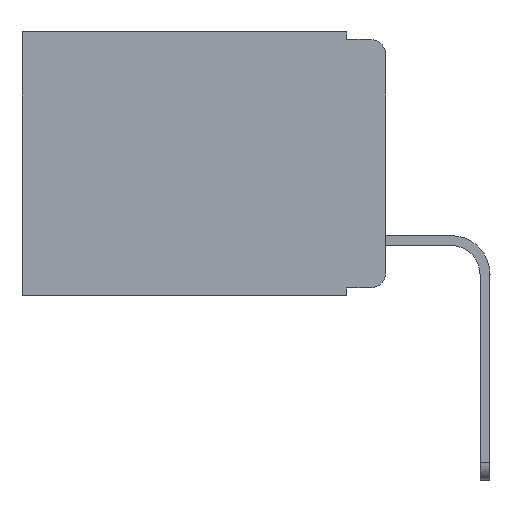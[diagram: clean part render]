
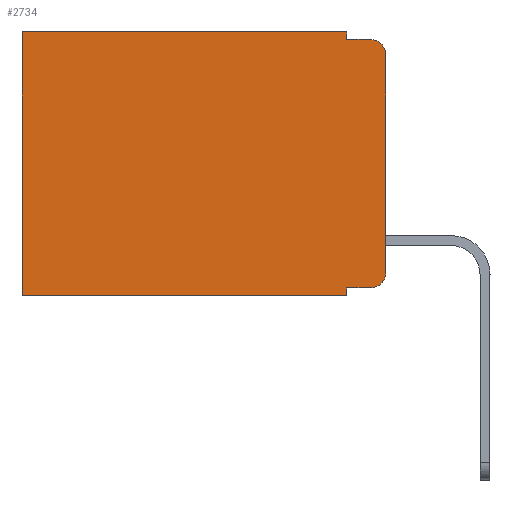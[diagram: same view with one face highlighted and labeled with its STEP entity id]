
A CAD part, left-side view. The second image highlights one B-rep face of the part: STEP entity #2734.
In plain terms, the highlighted planar face has unit normal (-1, 0, 0).
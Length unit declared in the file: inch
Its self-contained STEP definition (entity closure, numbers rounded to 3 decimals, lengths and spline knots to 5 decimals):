
#2 = VERTEX_POINT ( 'NONE', #6045 ) ;
#216 = ORIENTED_EDGE ( 'NONE', *, *, #6812, .T. ) ;
#849 = DIRECTION ( 'NONE',  ( 0., 0., -1. ) ) ;
#1429 = CARTESIAN_POINT ( 'NONE',  ( 0.298, 0., -0.343 ) ) ;
#1672 = ORIENTED_EDGE ( 'NONE', *, *, #20627, .F. ) ;
#1677 = EDGE_CURVE ( 'NONE', #11442, #16737, #12815, .T. ) ;
#1827 = CARTESIAN_POINT ( 'NONE',  ( 0.298, 0.02, -0.01 ) ) ;
#2053 = VECTOR ( 'NONE', #10447, 39.37008 ) ;
#2139 = EDGE_CURVE ( 'NONE', #8923, #5568, #7746, .T. ) ;
#2531 = DIRECTION ( 'NONE',  ( 1., 0., 0. ) ) ;
#2625 = EDGE_LOOP ( 'NONE', ( #8860, #216, #11828, #1672, #8557, #4596, #9044, #21511, #10805, #8913 ) ) ;
#2734 = ADVANCED_FACE ( 'NONE', ( #10842 ), #6238, .F. ) ;
#2928 = EDGE_CURVE ( 'NONE', #5576, #5568, #15015, .T. ) ;
#3239 = CIRCLE ( 'NONE', #4356, 0.02 ) ;
#3259 = DIRECTION ( 'NONE',  ( 0., 0., -1. ) ) ;
#3328 = CARTESIAN_POINT ( 'NONE',  ( 0.298, 0., 0. ) ) ;
#3614 = LINE ( 'NONE', #19214, #21034 ) ;
#4116 = VECTOR ( 'NONE', #17791, 39.37008 ) ;
#4356 = AXIS2_PLACEMENT_3D ( 'NONE', #10709, #19660, #8898 ) ;
#4442 = CARTESIAN_POINT ( 'NONE',  ( 0.298, 0.051, 0. ) ) ;
#4596 = ORIENTED_EDGE ( 'NONE', *, *, #2928, .T. ) ;
#4863 = CARTESIAN_POINT ( 'NONE',  ( 0.298, 0.051, -0.01 ) ) ;
#5568 = VERTEX_POINT ( 'NONE', #13558 ) ;
#5576 = VERTEX_POINT ( 'NONE', #17140 ) ;
#5787 = CARTESIAN_POINT ( 'NONE',  ( 0.298, 0., -0.313 ) ) ;
#6045 = CARTESIAN_POINT ( 'NONE',  ( 0.298, 0.02, -0.333 ) ) ;
#6064 = LINE ( 'NONE', #15897, #4116 ) ;
#6238 = PLANE ( 'NONE',  #8133 ) ;
#6788 = LINE ( 'NONE', #3328, #8819 ) ;
#6812 = EDGE_CURVE ( 'NONE', #12176, #16737, #13694, .T. ) ;
#7023 = VECTOR ( 'NONE', #15436, 39.37008 ) ;
#7746 = LINE ( 'NONE', #1429, #2053 ) ;
#8133 = AXIS2_PLACEMENT_3D ( 'NONE', #20401, #2531, #11401 ) ;
#8557 = ORIENTED_EDGE ( 'NONE', *, *, #9566, .T. ) ;
#8819 = VECTOR ( 'NONE', #17392, 39.37008 ) ;
#8860 = ORIENTED_EDGE ( 'NONE', *, *, #18945, .F. ) ;
#8898 = DIRECTION ( 'NONE',  ( 0., 0., -1. ) ) ;
#8913 = ORIENTED_EDGE ( 'NONE', *, *, #22862, .T. ) ;
#8923 = VERTEX_POINT ( 'NONE', #9932 ) ;
#9044 = ORIENTED_EDGE ( 'NONE', *, *, #2139, .F. ) ;
#9566 = EDGE_CURVE ( 'NONE', #18761, #5576, #6788, .T. ) ;
#9932 = CARTESIAN_POINT ( 'NONE',  ( 0.298, 0.051, -0.343 ) ) ;
#10447 = DIRECTION ( 'NONE',  ( 0., 1., 0. ) ) ;
#10579 = CARTESIAN_POINT ( 'NONE',  ( 0.298, 0.473, 0. ) ) ;
#10685 = CARTESIAN_POINT ( 'NONE',  ( 0.298, 0.02, -0.03 ) ) ;
#10709 = CARTESIAN_POINT ( 'NONE',  ( 0.298, 0.02, -0.313 ) ) ;
#10749 = DIRECTION ( 'NONE',  ( 0., -1., 0. ) ) ;
#10805 = ORIENTED_EDGE ( 'NONE', *, *, #19672, .T. ) ;
#10842 = FACE_OUTER_BOUND ( 'NONE', #2625, .T. ) ;
#10925 = VERTEX_POINT ( 'NONE', #11952 ) ;
#11081 = CARTESIAN_POINT ( 'NONE',  ( 0.298, 0.051, -0.01 ) ) ;
#11401 = DIRECTION ( 'NONE',  ( 0., 0., -1. ) ) ;
#11442 = VERTEX_POINT ( 'NONE', #11081 ) ;
#11828 = ORIENTED_EDGE ( 'NONE', *, *, #1677, .F. ) ;
#11866 = CARTESIAN_POINT ( 'NONE',  ( 0.298, 0.051, 0. ) ) ;
#11887 = LINE ( 'NONE', #14563, #16080 ) ;
#11952 = CARTESIAN_POINT ( 'NONE',  ( 0.298, 0.051, -0.333 ) ) ;
#12176 = VERTEX_POINT ( 'NONE', #18829 ) ;
#12323 = EDGE_CURVE ( 'NONE', #10925, #8923, #3614, .T. ) ;
#12815 = LINE ( 'NONE', #4863, #21795 ) ;
#13558 = CARTESIAN_POINT ( 'NONE',  ( 0.298, 0.473, -0.343 ) ) ;
#13694 = CIRCLE ( 'NONE', #13772, 0.02 ) ;
#13772 = AXIS2_PLACEMENT_3D ( 'NONE', #10685, #14120, #3259 ) ;
#14120 = DIRECTION ( 'NONE',  ( -1., 0., 0. ) ) ;
#14563 = CARTESIAN_POINT ( 'NONE',  ( 0.298, 0.051, -0.333 ) ) ;
#15015 = LINE ( 'NONE', #10579, #18970 ) ;
#15436 = DIRECTION ( 'NONE',  ( 0., 0., -1. ) ) ;
#15897 = CARTESIAN_POINT ( 'NONE',  ( 0.298, 0., 0. ) ) ;
#16080 = VECTOR ( 'NONE', #10749, 39.37008 ) ;
#16737 = VERTEX_POINT ( 'NONE', #1827 ) ;
#17140 = CARTESIAN_POINT ( 'NONE',  ( 0.298, 0.473, 0. ) ) ;
#17392 = DIRECTION ( 'NONE',  ( 0., 1., 0. ) ) ;
#17791 = DIRECTION ( 'NONE',  ( 0., 0., -1. ) ) ;
#18761 = VERTEX_POINT ( 'NONE', #4442 ) ;
#18829 = CARTESIAN_POINT ( 'NONE',  ( 0.298, 0., -0.03 ) ) ;
#18945 = EDGE_CURVE ( 'NONE', #12176, #21571, #6064, .T. ) ;
#18970 = VECTOR ( 'NONE', #20998, 39.37008 ) ;
#19214 = CARTESIAN_POINT ( 'NONE',  ( 0.298, 0.051, 0. ) ) ;
#19660 = DIRECTION ( 'NONE',  ( -1., 0., 0. ) ) ;
#19672 = EDGE_CURVE ( 'NONE', #10925, #2, #11887, .T. ) ;
#20401 = CARTESIAN_POINT ( 'NONE',  ( 0.298, 0., 0. ) ) ;
#20627 = EDGE_CURVE ( 'NONE', #18761, #11442, #23079, .T. ) ;
#20998 = DIRECTION ( 'NONE',  ( 0., 0., -1. ) ) ;
#21034 = VECTOR ( 'NONE', #849, 39.37008 ) ;
#21035 = DIRECTION ( 'NONE',  ( 0., -1., 0. ) ) ;
#21511 = ORIENTED_EDGE ( 'NONE', *, *, #12323, .F. ) ;
#21571 = VERTEX_POINT ( 'NONE', #5787 ) ;
#21795 = VECTOR ( 'NONE', #21035, 39.37008 ) ;
#22862 = EDGE_CURVE ( 'NONE', #2, #21571, #3239, .T. ) ;
#23079 = LINE ( 'NONE', #11866, #7023 ) ;
